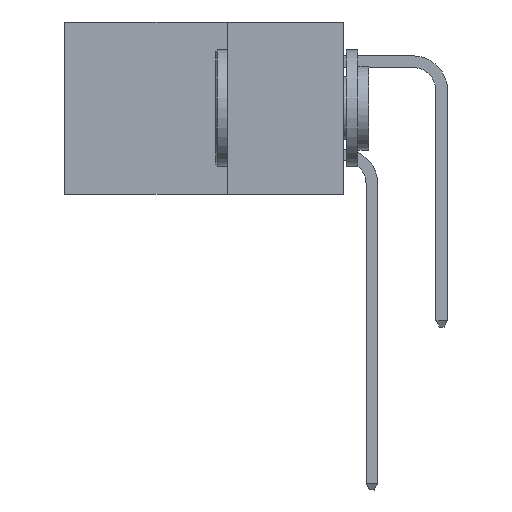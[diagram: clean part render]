
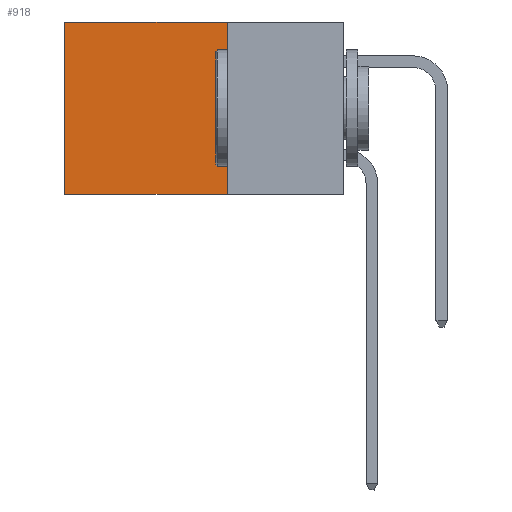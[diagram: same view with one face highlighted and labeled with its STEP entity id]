
A CAD part, left-side view. The second image highlights one B-rep face of the part: STEP entity #918.
In plain terms, the highlighted planar face has unit normal (-1, 0, 0).
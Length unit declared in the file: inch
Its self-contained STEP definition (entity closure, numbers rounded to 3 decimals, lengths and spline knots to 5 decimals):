
#587 = VECTOR ( 'NONE', #19769, 39.37008 ) ;
#623 = CARTESIAN_POINT ( 'NONE',  ( 0.2615, 0.25, 0. ) ) ;
#918 = ADVANCED_FACE ( 'NONE', ( #12559 ), #20209, .F. ) ;
#2338 = LINE ( 'NONE', #23502, #16222 ) ;
#2485 = DIRECTION ( 'NONE',  ( 0., 0., -1. ) ) ;
#2984 = AXIS2_PLACEMENT_3D ( 'NONE', #8509, #16455, #12066 ) ;
#3410 = DIRECTION ( 'NONE',  ( 0., 1., 0. ) ) ;
#4459 = VERTEX_POINT ( 'NONE', #15172 ) ;
#5661 = EDGE_CURVE ( 'NONE', #7062, #4459, #22295, .T. ) ;
#6302 = LINE ( 'NONE', #623, #587 ) ;
#7062 = VERTEX_POINT ( 'NONE', #10980 ) ;
#8169 = EDGE_LOOP ( 'NONE', ( #22063, #20147, #15445, #21390 ) ) ;
#8509 = CARTESIAN_POINT ( 'NONE',  ( 0.2615, 0.25, -0.37 ) ) ;
#10980 = CARTESIAN_POINT ( 'NONE',  ( 0.2615, 0.25, -0.37 ) ) ;
#11432 = CARTESIAN_POINT ( 'NONE',  ( 0.2615, 0.6, 0. ) ) ;
#12066 = DIRECTION ( 'NONE',  ( 0., 0., -1. ) ) ;
#12322 = LINE ( 'NONE', #21616, #16166 ) ;
#12559 = FACE_OUTER_BOUND ( 'NONE', #8169, .T. ) ;
#12917 = EDGE_CURVE ( 'NONE', #22319, #7062, #2338, .T. ) ;
#15172 = CARTESIAN_POINT ( 'NONE',  ( 0.2615, 0.6, -0.37 ) ) ;
#15445 = ORIENTED_EDGE ( 'NONE', *, *, #12917, .F. ) ;
#16166 = VECTOR ( 'NONE', #2485, 39.37008 ) ;
#16222 = VECTOR ( 'NONE', #17842, 39.37008 ) ;
#16455 = DIRECTION ( 'NONE',  ( 1., 0., 0. ) ) ;
#16657 = CARTESIAN_POINT ( 'NONE',  ( 0.2615, 0.25, -0.37 ) ) ;
#17842 = DIRECTION ( 'NONE',  ( 0., 0., -1. ) ) ;
#18072 = EDGE_CURVE ( 'NONE', #24334, #4459, #12322, .T. ) ;
#19769 = DIRECTION ( 'NONE',  ( 0., 1., 0. ) ) ;
#20147 = ORIENTED_EDGE ( 'NONE', *, *, #5661, .F. ) ;
#20209 = PLANE ( 'NONE',  #2984 ) ;
#21390 = ORIENTED_EDGE ( 'NONE', *, *, #22243, .T. ) ;
#21616 = CARTESIAN_POINT ( 'NONE',  ( 0.2615, 0.6, -0.37 ) ) ;
#22063 = ORIENTED_EDGE ( 'NONE', *, *, #18072, .T. ) ;
#22099 = VECTOR ( 'NONE', #3410, 39.37008 ) ;
#22243 = EDGE_CURVE ( 'NONE', #22319, #24334, #6302, .T. ) ;
#22295 = LINE ( 'NONE', #16657, #22099 ) ;
#22319 = VERTEX_POINT ( 'NONE', #23926 ) ;
#23502 = CARTESIAN_POINT ( 'NONE',  ( 0.2615, 0.25, -0.37 ) ) ;
#23926 = CARTESIAN_POINT ( 'NONE',  ( 0.2615, 0.25, 0. ) ) ;
#24334 = VERTEX_POINT ( 'NONE', #11432 ) ;
